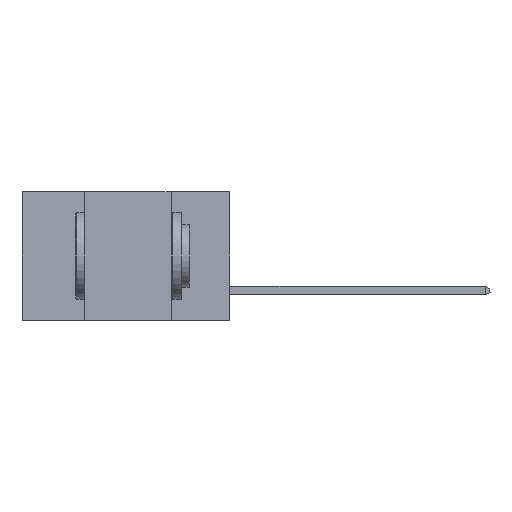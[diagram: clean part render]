
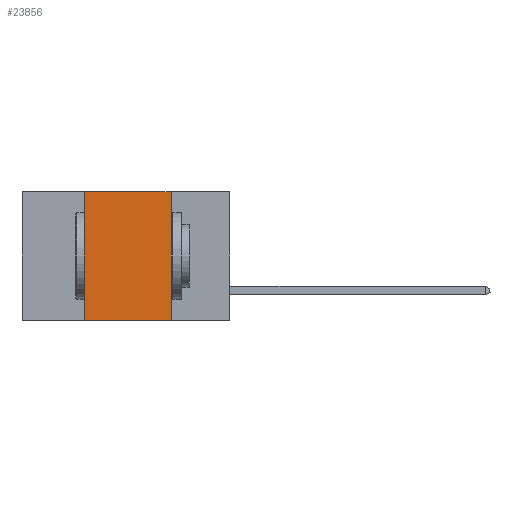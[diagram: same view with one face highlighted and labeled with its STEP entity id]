
A CAD part, left-side view. The second image highlights one B-rep face of the part: STEP entity #23856.
In plain terms, the highlighted planar face has unit normal (-1, 0, 0).
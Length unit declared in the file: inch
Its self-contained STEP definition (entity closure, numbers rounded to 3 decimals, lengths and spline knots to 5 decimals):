
#36 = FACE_OUTER_BOUND ( 'NONE', #18122, .T. ) ;
#224 = CARTESIAN_POINT ( 'NONE',  ( 0., 0.42, 0. ) ) ;
#1902 = CARTESIAN_POINT ( 'NONE',  ( 0., 0.6, 0. ) ) ;
#3132 = VECTOR ( 'NONE', #9073, 39.37008 ) ;
#4467 = VECTOR ( 'NONE', #15386, 39.37008 ) ;
#4578 = ORIENTED_EDGE ( 'NONE', *, *, #19426, .T. ) ;
#4749 = LINE ( 'NONE', #16237, #17750 ) ;
#5050 = CARTESIAN_POINT ( 'NONE',  ( 0., 0.6, -0.37 ) ) ;
#5169 = AXIS2_PLACEMENT_3D ( 'NONE', #15238, #19260, #5347 ) ;
#5234 = CARTESIAN_POINT ( 'NONE',  ( 0., 0.17, -0.37 ) ) ;
#5347 = DIRECTION ( 'NONE',  ( 0., 0., -1. ) ) ;
#5607 = EDGE_CURVE ( 'NONE', #17224, #8937, #24687, .T. ) ;
#6194 = CARTESIAN_POINT ( 'NONE',  ( 0., 0.17, 0. ) ) ;
#6777 = VERTEX_POINT ( 'NONE', #6194 ) ;
#8080 = ORIENTED_EDGE ( 'NONE', *, *, #24550, .F. ) ;
#8937 = VERTEX_POINT ( 'NONE', #224 ) ;
#9073 = DIRECTION ( 'NONE',  ( 0., 0., 1. ) ) ;
#9858 = LINE ( 'NONE', #5050, #4467 ) ;
#10400 = ORIENTED_EDGE ( 'NONE', *, *, #5607, .F. ) ;
#15238 = CARTESIAN_POINT ( 'NONE',  ( 0., 0.6, 0. ) ) ;
#15386 = DIRECTION ( 'NONE',  ( 0., -1., 0. ) ) ;
#15502 = PLANE ( 'NONE',  #5169 ) ;
#16237 = CARTESIAN_POINT ( 'NONE',  ( 0., 0.17, 0. ) ) ;
#17224 = VERTEX_POINT ( 'NONE', #18969 ) ;
#17750 = VECTOR ( 'NONE', #22325, 39.37008 ) ;
#18122 = EDGE_LOOP ( 'NONE', ( #8080, #25393, #10400, #4578 ) ) ;
#18529 = VECTOR ( 'NONE', #24921, 39.37008 ) ;
#18969 = CARTESIAN_POINT ( 'NONE',  ( 0., 0.42, -0.37 ) ) ;
#19152 = CARTESIAN_POINT ( 'NONE',  ( 0., 0.42, 0. ) ) ;
#19260 = DIRECTION ( 'NONE',  ( 1., 0., 0. ) ) ;
#19426 = EDGE_CURVE ( 'NONE', #17224, #24393, #9858, .T. ) ;
#20116 = LINE ( 'NONE', #1902, #18529 ) ;
#22126 = EDGE_CURVE ( 'NONE', #8937, #6777, #20116, .T. ) ;
#22325 = DIRECTION ( 'NONE',  ( 0., 0., -1. ) ) ;
#23856 = ADVANCED_FACE ( 'NONE', ( #36 ), #15502, .F. ) ;
#24393 = VERTEX_POINT ( 'NONE', #5234 ) ;
#24550 = EDGE_CURVE ( 'NONE', #6777, #24393, #4749, .T. ) ;
#24687 = LINE ( 'NONE', #19152, #3132 ) ;
#24921 = DIRECTION ( 'NONE',  ( 0., -1., 0. ) ) ;
#25393 = ORIENTED_EDGE ( 'NONE', *, *, #22126, .F. ) ;
